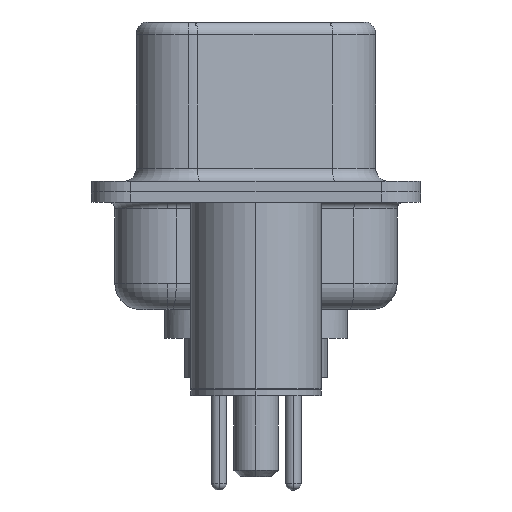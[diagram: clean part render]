
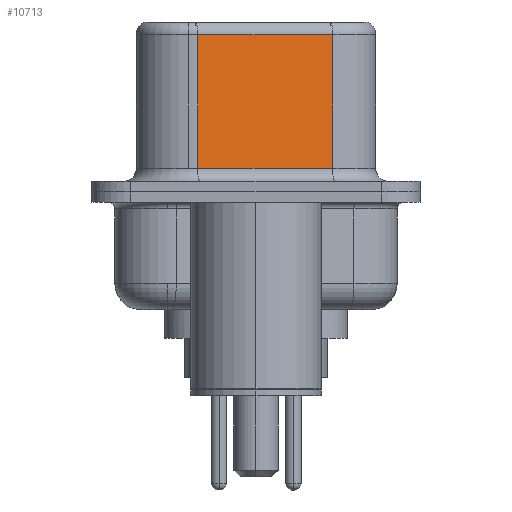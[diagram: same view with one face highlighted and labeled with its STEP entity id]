
A CAD part, left-side view. The second image highlights one B-rep face of the part: STEP entity #10713.
In plain terms, the highlighted planar face has unit normal (-0.985, -0.174, 0).
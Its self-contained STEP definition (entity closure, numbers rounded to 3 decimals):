
#105 = CARTESIAN_POINT ( 'NONE',  ( 4.58, -2.927, 0.9 ) ) ;
#539 = VERTEX_POINT ( 'NONE', #8440 ) ;
#1746 = CARTESIAN_POINT ( 'NONE',  ( 3.67, 2.233, 0.9 ) ) ;
#2211 = VECTOR ( 'NONE', #21854, 1000. ) ;
#2837 = DIRECTION ( 'NONE',  ( -0.174, 0.985, 0. ) ) ;
#3337 = VERTEX_POINT ( 'NONE', #22992 ) ;
#3381 = ORIENTED_EDGE ( 'NONE', *, *, #7886, .F. ) ;
#3502 = ORIENTED_EDGE ( 'NONE', *, *, #9137, .T. ) ;
#3917 = LINE ( 'NONE', #10839, #16956 ) ;
#4513 = CARTESIAN_POINT ( 'NONE',  ( 4.58, -2.927, 6.52 ) ) ;
#4559 = LINE ( 'NONE', #105, #13656 ) ;
#5321 = ORIENTED_EDGE ( 'NONE', *, *, #15850, .T. ) ;
#5954 = PLANE ( 'NONE',  #20234 ) ;
#6364 = FACE_OUTER_BOUND ( 'NONE', #10846, .T. ) ;
#7452 = DIRECTION ( 'NONE',  ( -0.174, 0.985, 0. ) ) ;
#7886 = EDGE_CURVE ( 'NONE', #15335, #539, #22638, .T. ) ;
#8440 = CARTESIAN_POINT ( 'NONE',  ( 4.58, -2.927, 0.9 ) ) ;
#9137 = EDGE_CURVE ( 'NONE', #3337, #18813, #15515, .T. ) ;
#10713 = ADVANCED_FACE ( 'NONE', ( #6364 ), #5954, .F. ) ;
#10839 = CARTESIAN_POINT ( 'NONE',  ( 4.58, -2.927, 6.02 ) ) ;
#10846 = EDGE_LOOP ( 'NONE', ( #3381, #5321, #3502, #19611 ) ) ;
#13316 = CARTESIAN_POINT ( 'NONE',  ( 3.67, 2.233, 6.52 ) ) ;
#13656 = VECTOR ( 'NONE', #21486, 1000. ) ;
#13724 = DIRECTION ( 'NONE',  ( 0.985, 0.174, 0. ) ) ;
#15243 = DIRECTION ( 'NONE',  ( 0., 0., -1. ) ) ;
#15335 = VERTEX_POINT ( 'NONE', #19642 ) ;
#15515 = LINE ( 'NONE', #13316, #22852 ) ;
#15850 = EDGE_CURVE ( 'NONE', #15335, #3337, #3917, .T. ) ;
#16956 = VECTOR ( 'NONE', #7452, 1000. ) ;
#17422 = EDGE_CURVE ( 'NONE', #18813, #539, #4559, .T. ) ;
#18813 = VERTEX_POINT ( 'NONE', #1746 ) ;
#19611 = ORIENTED_EDGE ( 'NONE', *, *, #17422, .T. ) ;
#19642 = CARTESIAN_POINT ( 'NONE',  ( 4.58, -2.927, 6.02 ) ) ;
#20234 = AXIS2_PLACEMENT_3D ( 'NONE', #4513, #13724, #2837 ) ;
#21486 = DIRECTION ( 'NONE',  ( 0.174, -0.985, 0. ) ) ;
#21854 = DIRECTION ( 'NONE',  ( 0., 0., -1. ) ) ;
#22165 = CARTESIAN_POINT ( 'NONE',  ( 4.58, -2.927, 6.52 ) ) ;
#22638 = LINE ( 'NONE', #22165, #2211 ) ;
#22852 = VECTOR ( 'NONE', #15243, 1000. ) ;
#22992 = CARTESIAN_POINT ( 'NONE',  ( 3.67, 2.233, 6.02 ) ) ;
